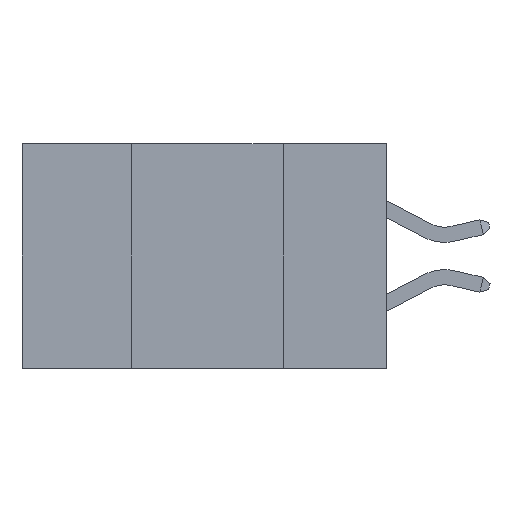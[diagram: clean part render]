
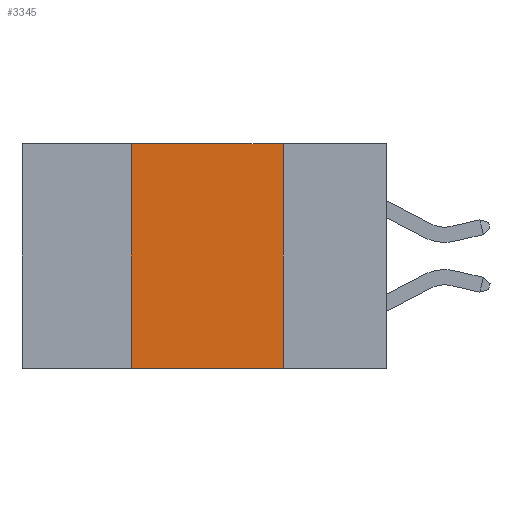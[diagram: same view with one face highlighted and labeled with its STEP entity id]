
A CAD part, left-side view. The second image highlights one B-rep face of the part: STEP entity #3345.
In plain terms, the highlighted planar face has unit normal (-1, 0, 0).
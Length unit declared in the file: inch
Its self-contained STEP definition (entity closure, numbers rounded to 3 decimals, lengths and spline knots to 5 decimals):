
#151 = CARTESIAN_POINT ( 'NONE',  ( 0., 0.6, 0. ) ) ;
#2360 = LINE ( 'NONE', #2902, #7210 ) ;
#2456 = DIRECTION ( 'NONE',  ( 0., 0., -1. ) ) ;
#2902 = CARTESIAN_POINT ( 'NONE',  ( 0., 0.17, 0. ) ) ;
#3345 = ADVANCED_FACE ( 'NONE', ( #15931 ), #15930, .F. ) ;
#3714 = CARTESIAN_POINT ( 'NONE',  ( 0., 0.42, 0. ) ) ;
#4359 = VERTEX_POINT ( 'NONE', #15020 ) ;
#4390 = LINE ( 'NONE', #3714, #9829 ) ;
#4534 = CARTESIAN_POINT ( 'NONE',  ( 0., 0.17, 0. ) ) ;
#4774 = CARTESIAN_POINT ( 'NONE',  ( 0., 0.6, 0. ) ) ;
#5253 = CARTESIAN_POINT ( 'NONE',  ( 0., 0.42, -0.37 ) ) ;
#5687 = EDGE_CURVE ( 'NONE', #8364, #4359, #4390, .T. ) ;
#6298 = DIRECTION ( 'NONE',  ( 0., -1., 0. ) ) ;
#7210 = VECTOR ( 'NONE', #7686, 39.37008 ) ;
#7593 = VECTOR ( 'NONE', #12632, 39.37008 ) ;
#7686 = DIRECTION ( 'NONE',  ( 0., 0., -1. ) ) ;
#7828 = ORIENTED_EDGE ( 'NONE', *, *, #16101, .T. ) ;
#8364 = VERTEX_POINT ( 'NONE', #5253 ) ;
#8558 = LINE ( 'NONE', #151, #12466 ) ;
#8926 = LINE ( 'NONE', #12295, #7593 ) ;
#9496 = DIRECTION ( 'NONE',  ( 1., 0., 0. ) ) ;
#9829 = VECTOR ( 'NONE', #13660, 39.37008 ) ;
#9866 = ORIENTED_EDGE ( 'NONE', *, *, #11438, .F. ) ;
#10347 = AXIS2_PLACEMENT_3D ( 'NONE', #4774, #9496, #2456 ) ;
#11438 = EDGE_CURVE ( 'NONE', #14548, #11648, #2360, .T. ) ;
#11648 = VERTEX_POINT ( 'NONE', #13353 ) ;
#12295 = CARTESIAN_POINT ( 'NONE',  ( 0., 0.6, -0.37 ) ) ;
#12466 = VECTOR ( 'NONE', #6298, 39.37008 ) ;
#12632 = DIRECTION ( 'NONE',  ( 0., -1., 0. ) ) ;
#13353 = CARTESIAN_POINT ( 'NONE',  ( 0., 0.17, -0.37 ) ) ;
#13551 = ORIENTED_EDGE ( 'NONE', *, *, #5687, .F. ) ;
#13660 = DIRECTION ( 'NONE',  ( 0., 0., 1. ) ) ;
#14507 = EDGE_LOOP ( 'NONE', ( #9866, #14618, #13551, #7828 ) ) ;
#14548 = VERTEX_POINT ( 'NONE', #4534 ) ;
#14618 = ORIENTED_EDGE ( 'NONE', *, *, #15374, .F. ) ;
#15020 = CARTESIAN_POINT ( 'NONE',  ( 0., 0.42, 0. ) ) ;
#15374 = EDGE_CURVE ( 'NONE', #4359, #14548, #8558, .T. ) ;
#15930 = PLANE ( 'NONE',  #10347 ) ;
#15931 = FACE_OUTER_BOUND ( 'NONE', #14507, .T. ) ;
#16101 = EDGE_CURVE ( 'NONE', #8364, #11648, #8926, .T. ) ;
